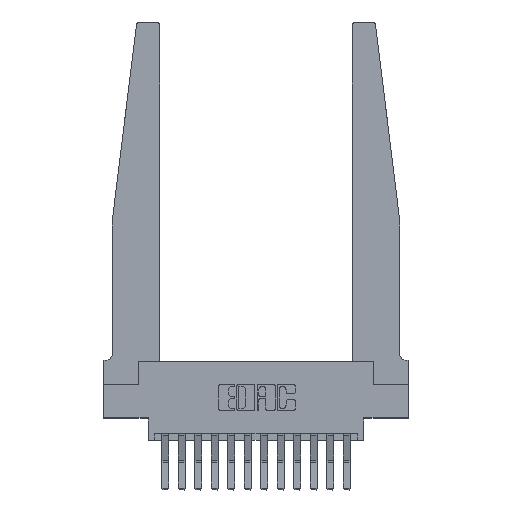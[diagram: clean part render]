
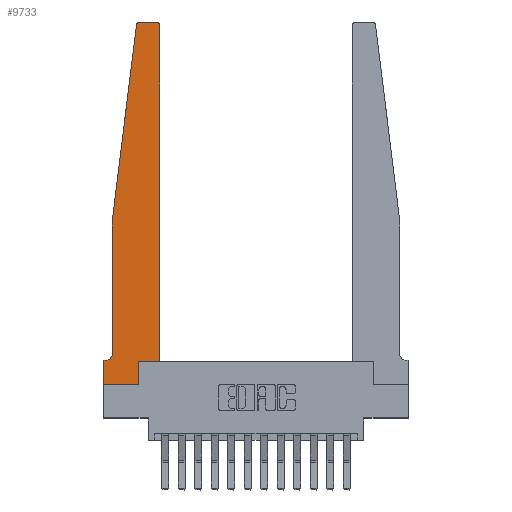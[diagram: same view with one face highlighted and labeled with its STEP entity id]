
A CAD part, top view. The second image highlights one B-rep face of the part: STEP entity #9733.
In plain terms, the highlighted planar face has unit normal (0, 0, 1).
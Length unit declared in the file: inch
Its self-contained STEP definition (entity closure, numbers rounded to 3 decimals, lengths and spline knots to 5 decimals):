
#136 = ORIENTED_EDGE ( 'NONE', *, *, #4102, .T. ) ;
#182 = CARTESIAN_POINT ( 'NONE',  ( 0.425, 2.72, 0.37 ) ) ;
#217 = ORIENTED_EDGE ( 'NONE', *, *, #15950, .T. ) ;
#285 = EDGE_CURVE ( 'NONE', #4407, #14129, #16675, .T. ) ;
#415 = DIRECTION ( 'NONE',  ( 0., -1., 0. ) ) ;
#667 = CARTESIAN_POINT ( 'NONE',  ( 0.065, 1.25, 0.37 ) ) ;
#677 = DIRECTION ( 'NONE',  ( -0.122, -0.992, 0. ) ) ;
#852 = FACE_OUTER_BOUND ( 'NONE', #11446, .T. ) ;
#946 = LINE ( 'NONE', #5068, #5611 ) ;
#1144 = LINE ( 'NONE', #11859, #1201 ) ;
#1201 = VECTOR ( 'NONE', #6452, 39.37008 ) ;
#1384 = VECTOR ( 'NONE', #6987, 39.37008 ) ;
#1543 = AXIS2_PLACEMENT_3D ( 'NONE', #1978, #13880, #11475 ) ;
#1670 = DIRECTION ( 'NONE',  ( -1., 0., 0. ) ) ;
#1797 = CARTESIAN_POINT ( 'NONE',  ( 0.425, 0.18, 0.37 ) ) ;
#1978 = CARTESIAN_POINT ( 'NONE',  ( 0., 0.1875, 0.37 ) ) ;
#2025 = CARTESIAN_POINT ( 'NONE',  ( 0., 0., 0.37 ) ) ;
#2245 = VECTOR ( 'NONE', #677, 39.37008 ) ;
#2387 = VERTEX_POINT ( 'NONE', #13422 ) ;
#3390 = ORIENTED_EDGE ( 'NONE', *, *, #7852, .T. ) ;
#3406 = DIRECTION ( 'NONE',  ( 0., 0., 1. ) ) ;
#3576 = CARTESIAN_POINT ( 'NONE',  ( 0.395, 2.72, 0.37 ) ) ;
#3873 = EDGE_CURVE ( 'NONE', #8896, #14956, #946, .T. ) ;
#3921 = DIRECTION ( 'NONE',  ( 0., 0., -1. ) ) ;
#4031 = VECTOR ( 'NONE', #415, 39.37008 ) ;
#4102 = EDGE_CURVE ( 'NONE', #14956, #7421, #1144, .T. ) ;
#4407 = VERTEX_POINT ( 'NONE', #14308 ) ;
#4595 = CARTESIAN_POINT ( 'NONE',  ( 0.2605, 0.18, 0.37 ) ) ;
#4781 = ORIENTED_EDGE ( 'NONE', *, *, #10395, .T. ) ;
#4925 = VERTEX_POINT ( 'NONE', #15409 ) ;
#4949 = EDGE_CURVE ( 'NONE', #2387, #17163, #14143, .T. ) ;
#5068 = CARTESIAN_POINT ( 'NONE',  ( 0.2605, 0.18, 0.37 ) ) ;
#5083 = LINE ( 'NONE', #9461, #8527 ) ;
#5129 = EDGE_CURVE ( 'NONE', #7421, #5629, #12632, .T. ) ;
#5611 = VECTOR ( 'NONE', #10529, 39.37008 ) ;
#5629 = VERTEX_POINT ( 'NONE', #182 ) ;
#6048 = ORIENTED_EDGE ( 'NONE', *, *, #9101, .T. ) ;
#6267 = DIRECTION ( 'NONE',  ( 1., 0., 0. ) ) ;
#6368 = CIRCLE ( 'NONE', #13081, 0.03 ) ;
#6452 = DIRECTION ( 'NONE',  ( 1., 0., 0. ) ) ;
#6881 = LINE ( 'NONE', #13718, #4031 ) ;
#6987 = DIRECTION ( 'NONE',  ( 1., 0., 0. ) ) ;
#7053 = VECTOR ( 'NONE', #9938, 39.37008 ) ;
#7210 = CIRCLE ( 'NONE', #16720, 0.03 ) ;
#7421 = VERTEX_POINT ( 'NONE', #17061 ) ;
#7466 = CARTESIAN_POINT ( 'NONE',  ( 0.27653, 2.72, 0.37 ) ) ;
#7654 = VECTOR ( 'NONE', #1670, 39.37008 ) ;
#7661 = ORIENTED_EDGE ( 'NONE', *, *, #15328, .T. ) ;
#7821 = CARTESIAN_POINT ( 'NONE',  ( 0.065, 0.1875, 0.37 ) ) ;
#7852 = EDGE_CURVE ( 'NONE', #4925, #12073, #10919, .T. ) ;
#8527 = VECTOR ( 'NONE', #10867, 39.37008 ) ;
#8687 = CARTESIAN_POINT ( 'NONE',  ( 0., 0.1875, 0.37 ) ) ;
#8896 = VERTEX_POINT ( 'NONE', #14649 ) ;
#8950 = EDGE_CURVE ( 'NONE', #11757, #2387, #9625, .T. ) ;
#9101 = EDGE_CURVE ( 'NONE', #17163, #14540, #6881, .T. ) ;
#9362 = LINE ( 'NONE', #9528, #1384 ) ;
#9461 = CARTESIAN_POINT ( 'NONE',  ( 0.065, 1.25, 0.37 ) ) ;
#9527 = CARTESIAN_POINT ( 'NONE',  ( 0.25, 2.75, 0.37 ) ) ;
#9528 = CARTESIAN_POINT ( 'NONE',  ( 0., 0., 0.37 ) ) ;
#9625 = CIRCLE ( 'NONE', #12121, 0.05 ) ;
#9733 = ADVANCED_FACE ( 'NONE', ( #852 ), #12542, .T. ) ;
#9938 = DIRECTION ( 'NONE',  ( 0., 1., 0. ) ) ;
#10395 = EDGE_CURVE ( 'NONE', #14129, #11757, #5083, .T. ) ;
#10529 = DIRECTION ( 'NONE',  ( 0., 1., 0. ) ) ;
#10582 = CARTESIAN_POINT ( 'NONE',  ( 0.015, 0.2375, 0.37 ) ) ;
#10751 = DIRECTION ( 'NONE',  ( -1., 0., 0. ) ) ;
#10867 = DIRECTION ( 'NONE',  ( 0., -1., 0. ) ) ;
#10919 = LINE ( 'NONE', #9527, #7654 ) ;
#11148 = CARTESIAN_POINT ( 'NONE',  ( 0.27653, 2.75, 0.37 ) ) ;
#11446 = EDGE_LOOP ( 'NONE', ( #3390, #7661, #12961, #4781, #14241, #11988, #6048, #217, #17207, #136, #12897, #16217 ) ) ;
#11475 = DIRECTION ( 'NONE',  ( 1., 0., 0. ) ) ;
#11757 = VERTEX_POINT ( 'NONE', #16988 ) ;
#11859 = CARTESIAN_POINT ( 'NONE',  ( 0.425, 0.18, 0.37 ) ) ;
#11988 = ORIENTED_EDGE ( 'NONE', *, *, #4949, .T. ) ;
#12073 = VERTEX_POINT ( 'NONE', #11148 ) ;
#12121 = AXIS2_PLACEMENT_3D ( 'NONE', #10582, #3921, #10751 ) ;
#12542 = PLANE ( 'NONE',  #1543 ) ;
#12632 = LINE ( 'NONE', #1797, #7053 ) ;
#12897 = ORIENTED_EDGE ( 'NONE', *, *, #5129, .T. ) ;
#12961 = ORIENTED_EDGE ( 'NONE', *, *, #285, .T. ) ;
#13081 = AXIS2_PLACEMENT_3D ( 'NONE', #7466, #16961, #6267 ) ;
#13422 = CARTESIAN_POINT ( 'NONE',  ( 0.015, 0.1875, 0.37 ) ) ;
#13480 = EDGE_CURVE ( 'NONE', #5629, #4925, #7210, .T. ) ;
#13718 = CARTESIAN_POINT ( 'NONE',  ( 0., 0., 0.37 ) ) ;
#13880 = DIRECTION ( 'NONE',  ( 0., 0., 1. ) ) ;
#14087 = DIRECTION ( 'NONE',  ( 1., 0., 0. ) ) ;
#14129 = VERTEX_POINT ( 'NONE', #667 ) ;
#14143 = LINE ( 'NONE', #7821, #16559 ) ;
#14216 = CARTESIAN_POINT ( 'NONE',  ( 0.065, 1.25, 0.37 ) ) ;
#14241 = ORIENTED_EDGE ( 'NONE', *, *, #8950, .T. ) ;
#14308 = CARTESIAN_POINT ( 'NONE',  ( 0.24675, 2.72367, 0.37 ) ) ;
#14540 = VERTEX_POINT ( 'NONE', #2025 ) ;
#14649 = CARTESIAN_POINT ( 'NONE',  ( 0.2605, 0., 0.37 ) ) ;
#14956 = VERTEX_POINT ( 'NONE', #4595 ) ;
#15328 = EDGE_CURVE ( 'NONE', #12073, #4407, #6368, .T. ) ;
#15409 = CARTESIAN_POINT ( 'NONE',  ( 0.395, 2.75, 0.37 ) ) ;
#15475 = DIRECTION ( 'NONE',  ( -1., 0., 0. ) ) ;
#15950 = EDGE_CURVE ( 'NONE', #14540, #8896, #9362, .T. ) ;
#16217 = ORIENTED_EDGE ( 'NONE', *, *, #13480, .T. ) ;
#16559 = VECTOR ( 'NONE', #15475, 39.37008 ) ;
#16675 = LINE ( 'NONE', #14216, #2245 ) ;
#16720 = AXIS2_PLACEMENT_3D ( 'NONE', #3576, #3406, #14087 ) ;
#16961 = DIRECTION ( 'NONE',  ( 0., 0., 1. ) ) ;
#16988 = CARTESIAN_POINT ( 'NONE',  ( 0.065, 0.2375, 0.37 ) ) ;
#17061 = CARTESIAN_POINT ( 'NONE',  ( 0.425, 0.18, 0.37 ) ) ;
#17163 = VERTEX_POINT ( 'NONE', #8687 ) ;
#17207 = ORIENTED_EDGE ( 'NONE', *, *, #3873, .T. ) ;
